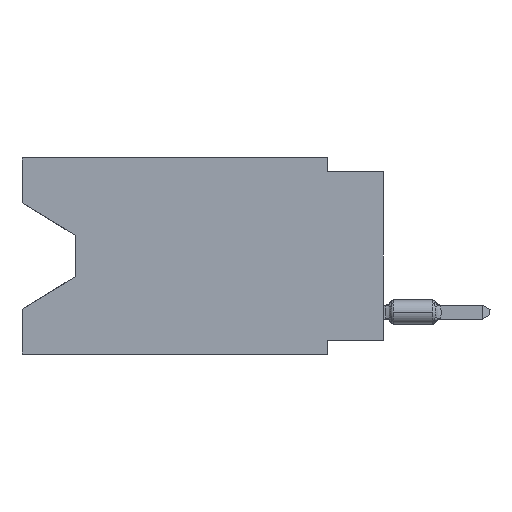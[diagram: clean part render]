
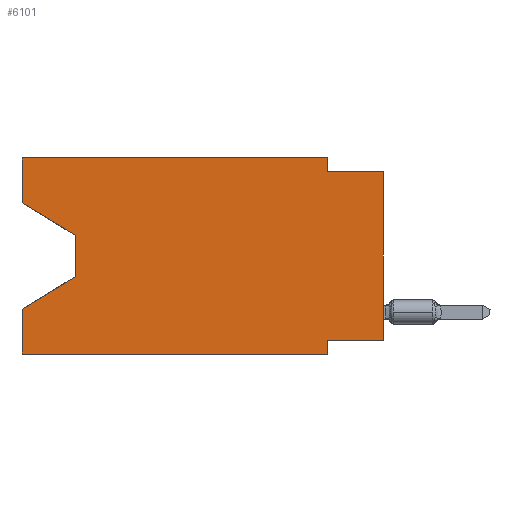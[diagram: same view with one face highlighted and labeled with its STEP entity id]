
A CAD part, left-side view. The second image highlights one B-rep face of the part: STEP entity #6101.
In plain terms, the highlighted planar face has unit normal (-1, 0, 0).
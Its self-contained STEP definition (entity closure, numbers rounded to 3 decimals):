
#157 = VERTEX_POINT ( 'NONE', #20666 ) ;
#177 = CARTESIAN_POINT ( 'NONE',  ( 0., 0., 0. ) ) ;
#569 = DIRECTION ( 'NONE',  ( 0., 0., -1. ) ) ;
#1093 = CARTESIAN_POINT ( 'NONE',  ( 0., 0., -8.255 ) ) ;
#1282 = VERTEX_POINT ( 'NONE', #1093 ) ;
#1388 = CARTESIAN_POINT ( 'NONE',  ( 0., 0., -0.635 ) ) ;
#1486 = DIRECTION ( 'NONE',  ( 0., 0., 1. ) ) ;
#1515 = ORIENTED_EDGE ( 'NONE', *, *, #8024, .F. ) ;
#1736 = VECTOR ( 'NONE', #14939, 1000. ) ;
#1986 = LINE ( 'NONE', #5458, #16236 ) ;
#2426 = CARTESIAN_POINT ( 'NONE',  ( 0., 2.54, 0. ) ) ;
#2514 = CARTESIAN_POINT ( 'NONE',  ( 0., 16.383, -8.89 ) ) ;
#2529 = DIRECTION ( 'NONE',  ( 0., 0., 1. ) ) ;
#2633 = VERTEX_POINT ( 'NONE', #7360 ) ;
#2843 = VERTEX_POINT ( 'NONE', #18754 ) ;
#4094 = VERTEX_POINT ( 'NONE', #22766 ) ;
#4339 = DIRECTION ( 'NONE',  ( 0., 0.855, -0.519 ) ) ;
#4421 = CARTESIAN_POINT ( 'NONE',  ( 0., 16.383, 0. ) ) ;
#4427 = AXIS2_PLACEMENT_3D ( 'NONE', #11639, #18662, #569 ) ;
#4531 = ORIENTED_EDGE ( 'NONE', *, *, #11794, .F. ) ;
#4617 = PLANE ( 'NONE',  #4427 ) ;
#4640 = LINE ( 'NONE', #4421, #18189 ) ;
#4849 = CARTESIAN_POINT ( 'NONE',  ( 0., 2.54, -0.635 ) ) ;
#5092 = EDGE_CURVE ( 'NONE', #12000, #4094, #14972, .T. ) ;
#5428 = EDGE_CURVE ( 'NONE', #2843, #11775, #11588, .T. ) ;
#5458 = CARTESIAN_POINT ( 'NONE',  ( 0., 2.54, -8.89 ) ) ;
#5590 = ORIENTED_EDGE ( 'NONE', *, *, #7849, .T. ) ;
#5801 = ORIENTED_EDGE ( 'NONE', *, *, #14197, .T. ) ;
#5838 = LINE ( 'NONE', #18268, #8704 ) ;
#5907 = DIRECTION ( 'NONE',  ( 0., 0., -1. ) ) ;
#6101 = ADVANCED_FACE ( 'NONE', ( #13270 ), #4617, .F. ) ;
#6272 = VECTOR ( 'NONE', #5907, 1000. ) ;
#6446 = LINE ( 'NONE', #22117, #7310 ) ;
#6601 = CARTESIAN_POINT ( 'NONE',  ( 0., 16.383, -2.038 ) ) ;
#6625 = LINE ( 'NONE', #16768, #17134 ) ;
#6667 = ORIENTED_EDGE ( 'NONE', *, *, #21173, .T. ) ;
#7310 = VECTOR ( 'NONE', #8066, 1000. ) ;
#7360 = CARTESIAN_POINT ( 'NONE',  ( 0., 2.54, -8.89 ) ) ;
#7849 = EDGE_CURVE ( 'NONE', #12952, #2843, #6446, .T. ) ;
#7873 = ORIENTED_EDGE ( 'NONE', *, *, #15404, .F. ) ;
#8024 = EDGE_CURVE ( 'NONE', #12952, #13078, #11866, .T. ) ;
#8066 = DIRECTION ( 'NONE',  ( 0., -0.855, -0.519 ) ) ;
#8704 = VECTOR ( 'NONE', #4339, 1000. ) ;
#8847 = ORIENTED_EDGE ( 'NONE', *, *, #21505, .F. ) ;
#9653 = DIRECTION ( 'NONE',  ( 0., 0., -1. ) ) ;
#9852 = EDGE_CURVE ( 'NONE', #1282, #19003, #19429, .T. ) ;
#10164 = CARTESIAN_POINT ( 'NONE',  ( 0., 16.383, 0. ) ) ;
#10259 = EDGE_LOOP ( 'NONE', ( #5590, #21652, #5801, #14109, #6667, #19153, #22281, #19137, #7873, #8847, #4531, #1515 ) ) ;
#10516 = VERTEX_POINT ( 'NONE', #4849 ) ;
#11069 = VECTOR ( 'NONE', #21257, 1000. ) ;
#11350 = EDGE_CURVE ( 'NONE', #1282, #157, #6625, .T. ) ;
#11588 = LINE ( 'NONE', #16906, #15077 ) ;
#11639 = CARTESIAN_POINT ( 'NONE',  ( 0., 16.383, 0. ) ) ;
#11775 = VERTEX_POINT ( 'NONE', #12605 ) ;
#11794 = EDGE_CURVE ( 'NONE', #13078, #21094, #4640, .T. ) ;
#11866 = LINE ( 'NONE', #17389, #16465 ) ;
#12000 = VERTEX_POINT ( 'NONE', #2514 ) ;
#12605 = CARTESIAN_POINT ( 'NONE',  ( 0., 13.97, -5.385 ) ) ;
#12907 = VECTOR ( 'NONE', #14122, 1000. ) ;
#12952 = VERTEX_POINT ( 'NONE', #6601 ) ;
#13078 = VERTEX_POINT ( 'NONE', #10164 ) ;
#13206 = DIRECTION ( 'NONE',  ( 0., 1., 0. ) ) ;
#13270 = FACE_OUTER_BOUND ( 'NONE', #10259, .T. ) ;
#14109 = ORIENTED_EDGE ( 'NONE', *, *, #5092, .F. ) ;
#14122 = DIRECTION ( 'NONE',  ( 0., -1., 0. ) ) ;
#14197 = EDGE_CURVE ( 'NONE', #11775, #4094, #5838, .T. ) ;
#14717 = LINE ( 'NONE', #18398, #1736 ) ;
#14939 = DIRECTION ( 'NONE',  ( 0., -1., 0. ) ) ;
#14972 = LINE ( 'NONE', #21985, #16213 ) ;
#15019 = DIRECTION ( 'NONE',  ( 0., -1., 0. ) ) ;
#15077 = VECTOR ( 'NONE', #9653, 1000. ) ;
#15124 = LINE ( 'NONE', #2426, #6272 ) ;
#15404 = EDGE_CURVE ( 'NONE', #10516, #19003, #14717, .T. ) ;
#15740 = CARTESIAN_POINT ( 'NONE',  ( 0., 16.383, -8.89 ) ) ;
#15940 = DIRECTION ( 'NONE',  ( 0., 0., -1. ) ) ;
#16213 = VECTOR ( 'NONE', #2529, 1000. ) ;
#16236 = VECTOR ( 'NONE', #15940, 1000. ) ;
#16465 = VECTOR ( 'NONE', #1486, 1000. ) ;
#16768 = CARTESIAN_POINT ( 'NONE',  ( 0., 0., -8.255 ) ) ;
#16906 = CARTESIAN_POINT ( 'NONE',  ( 0., 13.97, -3.505 ) ) ;
#17134 = VECTOR ( 'NONE', #13206, 1000. ) ;
#17389 = CARTESIAN_POINT ( 'NONE',  ( 0., 16.383, 0. ) ) ;
#17580 = CARTESIAN_POINT ( 'NONE',  ( 0., 2.54, 0. ) ) ;
#18189 = VECTOR ( 'NONE', #15019, 1000. ) ;
#18268 = CARTESIAN_POINT ( 'NONE',  ( 0., 13.97, -5.385 ) ) ;
#18398 = CARTESIAN_POINT ( 'NONE',  ( 0., 0., -0.635 ) ) ;
#18662 = DIRECTION ( 'NONE',  ( 1., 0., 0. ) ) ;
#18754 = CARTESIAN_POINT ( 'NONE',  ( 0., 13.97, -3.505 ) ) ;
#19003 = VERTEX_POINT ( 'NONE', #1388 ) ;
#19137 = ORIENTED_EDGE ( 'NONE', *, *, #9852, .T. ) ;
#19153 = ORIENTED_EDGE ( 'NONE', *, *, #22352, .F. ) ;
#19429 = LINE ( 'NONE', #177, #11069 ) ;
#20666 = CARTESIAN_POINT ( 'NONE',  ( 0., 2.54, -8.255 ) ) ;
#21094 = VERTEX_POINT ( 'NONE', #17580 ) ;
#21173 = EDGE_CURVE ( 'NONE', #12000, #2633, #21372, .T. ) ;
#21257 = DIRECTION ( 'NONE',  ( 0., 0., 1. ) ) ;
#21372 = LINE ( 'NONE', #15740, #12907 ) ;
#21505 = EDGE_CURVE ( 'NONE', #21094, #10516, #15124, .T. ) ;
#21652 = ORIENTED_EDGE ( 'NONE', *, *, #5428, .T. ) ;
#21985 = CARTESIAN_POINT ( 'NONE',  ( 0., 16.383, 0. ) ) ;
#22117 = CARTESIAN_POINT ( 'NONE',  ( 0., 16.383, -2.038 ) ) ;
#22281 = ORIENTED_EDGE ( 'NONE', *, *, #11350, .F. ) ;
#22352 = EDGE_CURVE ( 'NONE', #157, #2633, #1986, .T. ) ;
#22766 = CARTESIAN_POINT ( 'NONE',  ( 0., 16.383, -6.852 ) ) ;
